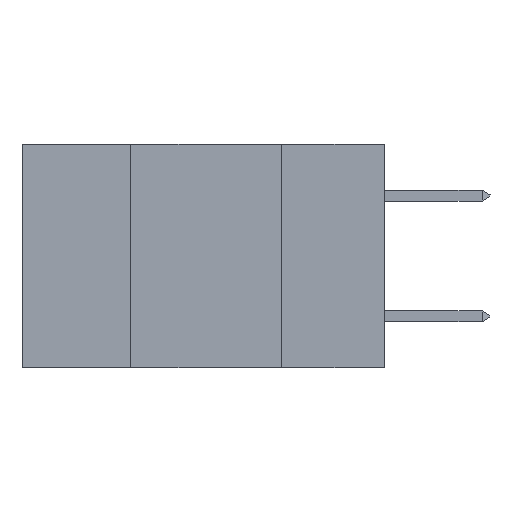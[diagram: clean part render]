
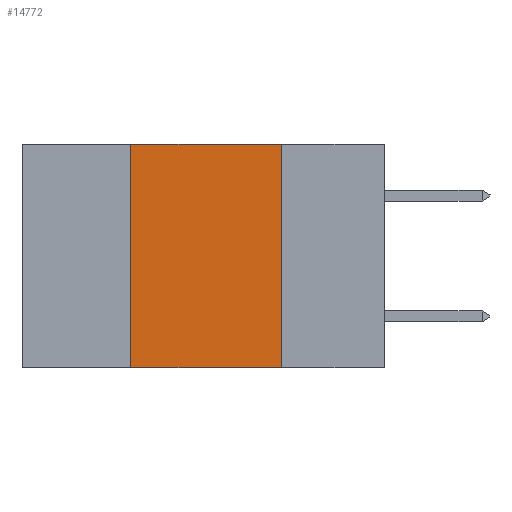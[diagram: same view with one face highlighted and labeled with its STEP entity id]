
A CAD part, left-side view. The second image highlights one B-rep face of the part: STEP entity #14772.
In plain terms, the highlighted planar face has unit normal (-1, 0, 0).
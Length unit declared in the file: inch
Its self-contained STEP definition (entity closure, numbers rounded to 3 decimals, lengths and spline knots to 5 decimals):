
#1278 = EDGE_CURVE ( 'NONE', #22428, #10768, #18268, .T. ) ;
#1944 = DIRECTION ( 'NONE',  ( 0., 0., -1. ) ) ;
#2143 = EDGE_CURVE ( 'NONE', #10768, #19536, #35448, .T. ) ;
#2651 = VECTOR ( 'NONE', #25880, 39.37008 ) ;
#2793 = CARTESIAN_POINT ( 'NONE',  ( 0., 0.6, -0.37 ) ) ;
#3763 = EDGE_CURVE ( 'NONE', #22428, #21150, #41901, .T. ) ;
#5673 = PLANE ( 'NONE',  #24827 ) ;
#9170 = CARTESIAN_POINT ( 'NONE',  ( 0., 0.17, 0. ) ) ;
#9444 = LINE ( 'NONE', #37318, #34939 ) ;
#10768 = VERTEX_POINT ( 'NONE', #26864 ) ;
#12573 = ORIENTED_EDGE ( 'NONE', *, *, #3763, .T. ) ;
#14291 = ORIENTED_EDGE ( 'NONE', *, *, #37831, .F. ) ;
#14772 = ADVANCED_FACE ( 'NONE', ( #24507 ), #5673, .F. ) ;
#14941 = DIRECTION ( 'NONE',  ( 0., -1., 0. ) ) ;
#15076 = DIRECTION ( 'NONE',  ( 1., 0., 0. ) ) ;
#18268 = LINE ( 'NONE', #28212, #22331 ) ;
#18651 = CARTESIAN_POINT ( 'NONE',  ( 0., 0.42, -0.37 ) ) ;
#18755 = ORIENTED_EDGE ( 'NONE', *, *, #2143, .F. ) ;
#19536 = VERTEX_POINT ( 'NONE', #9170 ) ;
#20134 = CARTESIAN_POINT ( 'NONE',  ( 0., 0.17, -0.37 ) ) ;
#21150 = VERTEX_POINT ( 'NONE', #20134 ) ;
#21539 = CARTESIAN_POINT ( 'NONE',  ( 0., 0.6, 0. ) ) ;
#22331 = VECTOR ( 'NONE', #38079, 39.37008 ) ;
#22428 = VERTEX_POINT ( 'NONE', #18651 ) ;
#24507 = FACE_OUTER_BOUND ( 'NONE', #27889, .T. ) ;
#24827 = AXIS2_PLACEMENT_3D ( 'NONE', #38179, #15076, #1944 ) ;
#25880 = DIRECTION ( 'NONE',  ( 0., -1., 0. ) ) ;
#26864 = CARTESIAN_POINT ( 'NONE',  ( 0., 0.42, 0. ) ) ;
#27889 = EDGE_LOOP ( 'NONE', ( #14291, #18755, #32733, #12573 ) ) ;
#28212 = CARTESIAN_POINT ( 'NONE',  ( 0., 0.42, 0. ) ) ;
#32733 = ORIENTED_EDGE ( 'NONE', *, *, #1278, .F. ) ;
#34939 = VECTOR ( 'NONE', #36903, 39.37008 ) ;
#35448 = LINE ( 'NONE', #21539, #38549 ) ;
#36903 = DIRECTION ( 'NONE',  ( 0., 0., -1. ) ) ;
#37318 = CARTESIAN_POINT ( 'NONE',  ( 0., 0.17, 0. ) ) ;
#37831 = EDGE_CURVE ( 'NONE', #19536, #21150, #9444, .T. ) ;
#38079 = DIRECTION ( 'NONE',  ( 0., 0., 1. ) ) ;
#38179 = CARTESIAN_POINT ( 'NONE',  ( 0., 0.6, 0. ) ) ;
#38549 = VECTOR ( 'NONE', #14941, 39.37008 ) ;
#41901 = LINE ( 'NONE', #2793, #2651 ) ;
